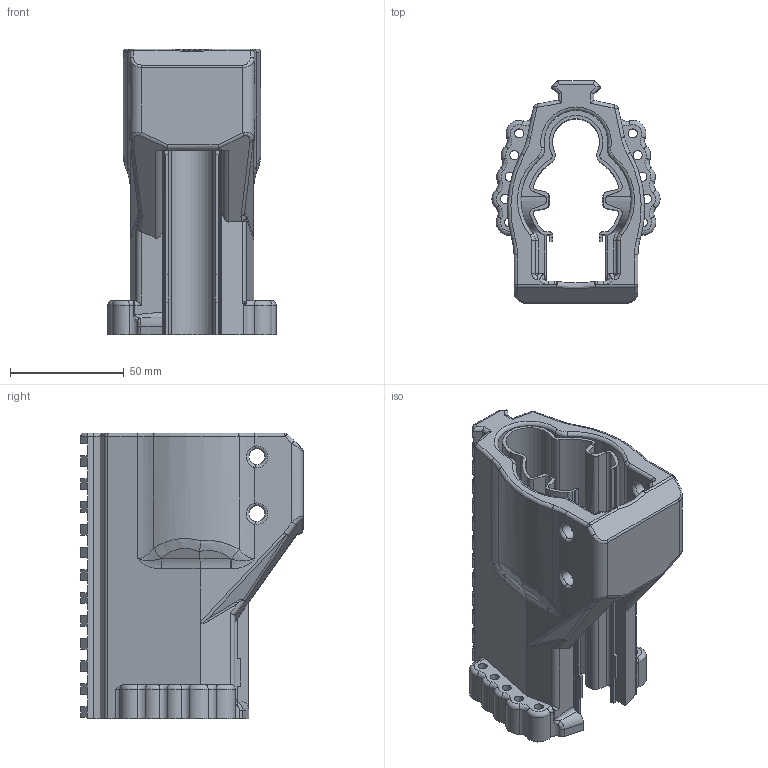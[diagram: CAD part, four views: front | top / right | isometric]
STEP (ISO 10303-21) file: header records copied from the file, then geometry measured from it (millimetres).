
FILE_DESCRIPTION(/* description */ (''),/* implementation_level */ '2;1');
FILE_NAME(/* name */ 'Rear Receiver Rev3.stp',/* time_stamp */ '2021-11-22T21:42:52-06:00',/* author */ ('johne'),/* organization */ (''),/* preprocessor_version */ 'ST-DEVELOPER v18.1',/* originating_system */ 'Autodesk Inventor 2020',/* authorisation */ '');
FILE_SCHEMA (('AUTOMOTIVE_DESIGN { 1 0 10303 214 3 1 1 }'));
Length unit declared in the file: inch
Products named in the file (1): Rear Receiver
Bounding box: 73.79 x 97.63 x 125.41 mm (x, y, z)
Volume: 258441.3 mm3; surface area: 73322.9 mm2
Topology: 1 solids, 1 shells, 423 faces, 1149 edges, 712 vertices
Faces by surface type: cylinder 158, plane 156, torus 58, bspline 43, sphere 8
Full cylindrical faces by diameter (mm): 4 x10, 7 x4
Entity records: 14821 total; most frequent: CARTESIAN_POINT 3973, DIRECTION 2293, ORIENTED_EDGE 2278, EDGE_CURVE 1139, AXIS2_PLACEMENT_3D 843, VERTEX_POINT 712, LINE 607, VECTOR 607
